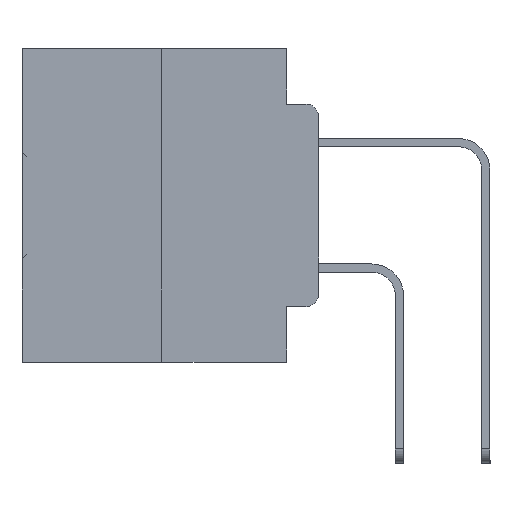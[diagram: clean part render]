
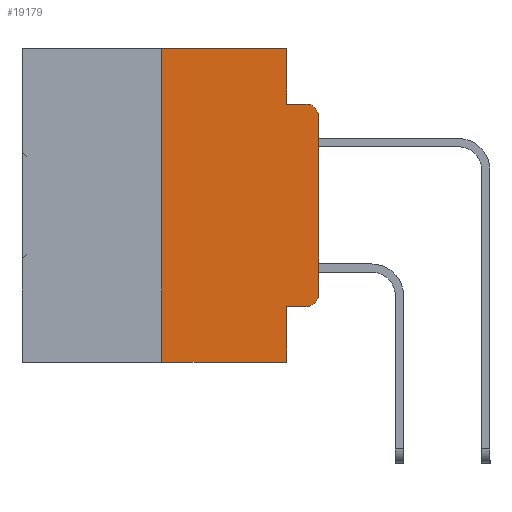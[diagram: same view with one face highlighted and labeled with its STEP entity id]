
A CAD part, left-side view. The second image highlights one B-rep face of the part: STEP entity #19179.
In plain terms, the highlighted planar face has unit normal (-1, 0, 0).
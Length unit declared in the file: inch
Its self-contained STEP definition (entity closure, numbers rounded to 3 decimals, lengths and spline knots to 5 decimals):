
#192 = ORIENTED_EDGE ( 'NONE', *, *, #10469, .T. ) ;
#581 = DIRECTION ( 'NONE',  ( 0., 0., -1. ) ) ;
#603 = ORIENTED_EDGE ( 'NONE', *, *, #27473, .F. ) ;
#792 = VECTOR ( 'NONE', #25249, 39.37008 ) ;
#964 = EDGE_CURVE ( 'NONE', #31384, #4274, #8654, .T. ) ;
#2047 = CARTESIAN_POINT ( 'NONE',  ( 0., 0.473, 0. ) ) ;
#2244 = CARTESIAN_POINT ( 'NONE',  ( 0., 0.473, 0. ) ) ;
#3590 = CARTESIAN_POINT ( 'NONE',  ( 0., 0., -0.3915 ) ) ;
#4274 = VERTEX_POINT ( 'NONE', #27666 ) ;
#4301 = AXIS2_PLACEMENT_3D ( 'NONE', #8759, #27886, #11510 ) ;
#4470 = CARTESIAN_POINT ( 'NONE',  ( 0., 0., 0. ) ) ;
#5002 = DIRECTION ( 'NONE',  ( 0., 0., -1. ) ) ;
#5069 = VERTEX_POINT ( 'NONE', #6417 ) ;
#6417 = CARTESIAN_POINT ( 'NONE',  ( 0., 0., -0.1085 ) ) ;
#7457 = CARTESIAN_POINT ( 'NONE',  ( 0., 0.051, 0. ) ) ;
#7655 = PLANE ( 'NONE',  #8157 ) ;
#8157 = AXIS2_PLACEMENT_3D ( 'NONE', #2244, #21437, #5002 ) ;
#8607 = VECTOR ( 'NONE', #19148, 39.37008 ) ;
#8654 = LINE ( 'NONE', #16856, #23241 ) ;
#8759 = CARTESIAN_POINT ( 'NONE',  ( 0., 0.02, -0.1085 ) ) ;
#9177 = LINE ( 'NONE', #33287, #22912 ) ;
#9994 = VECTOR ( 'NONE', #12510, 39.37008 ) ;
#10026 = ORIENTED_EDGE ( 'NONE', *, *, #31907, .T. ) ;
#10469 = EDGE_CURVE ( 'NONE', #33555, #27536, #14412, .T. ) ;
#10687 = CARTESIAN_POINT ( 'NONE',  ( 0., 0.25, 0. ) ) ;
#11510 = DIRECTION ( 'NONE',  ( 0., 0., -1. ) ) ;
#11627 = CARTESIAN_POINT ( 'NONE',  ( 0., 0.051, -0.4115 ) ) ;
#12165 = EDGE_CURVE ( 'NONE', #5069, #17493, #23960, .T. ) ;
#12510 = DIRECTION ( 'NONE',  ( 0., 0., 1. ) ) ;
#12594 = DIRECTION ( 'NONE',  ( -1., 0., 0. ) ) ;
#13788 = DIRECTION ( 'NONE',  ( 0., 0., -1. ) ) ;
#13917 = AXIS2_PLACEMENT_3D ( 'NONE', #28972, #12594, #31649 ) ;
#14412 = CIRCLE ( 'NONE', #13917, 0.02 ) ;
#15363 = VECTOR ( 'NONE', #19749, 39.37008 ) ;
#16356 = CARTESIAN_POINT ( 'NONE',  ( 0., 0.02, -0.0885 ) ) ;
#16700 = VERTEX_POINT ( 'NONE', #7457 ) ;
#16819 = FACE_OUTER_BOUND ( 'NONE', #20377, .T. ) ;
#16856 = CARTESIAN_POINT ( 'NONE',  ( 0., 0.473, -0.5 ) ) ;
#16872 = ORIENTED_EDGE ( 'NONE', *, *, #31974, .F. ) ;
#16901 = EDGE_CURVE ( 'NONE', #16700, #27307, #29192, .T. ) ;
#17063 = LINE ( 'NONE', #11627, #15363 ) ;
#17280 = VERTEX_POINT ( 'NONE', #26335 ) ;
#17318 = ORIENTED_EDGE ( 'NONE', *, *, #20610, .F. ) ;
#17493 = VERTEX_POINT ( 'NONE', #16356 ) ;
#19148 = DIRECTION ( 'NONE',  ( 0., 0., 1. ) ) ;
#19179 = ADVANCED_FACE ( 'NONE', ( #16819 ), #7655, .F. ) ;
#19429 = ORIENTED_EDGE ( 'NONE', *, *, #12165, .T. ) ;
#19490 = ORIENTED_EDGE ( 'NONE', *, *, #21764, .T. ) ;
#19749 = DIRECTION ( 'NONE',  ( 0., -1., 0. ) ) ;
#19907 = ORIENTED_EDGE ( 'NONE', *, *, #964, .T. ) ;
#20377 = EDGE_LOOP ( 'NONE', ( #10026, #19429, #26325, #25924, #16872, #17318, #19907, #603, #19490, #192 ) ) ;
#20544 = CARTESIAN_POINT ( 'NONE',  ( 0., 0.25, 0. ) ) ;
#20610 = EDGE_CURVE ( 'NONE', #31384, #27333, #30412, .T. ) ;
#21304 = EDGE_CURVE ( 'NONE', #27307, #17493, #22713, .T. ) ;
#21437 = DIRECTION ( 'NONE',  ( 1., 0., 0. ) ) ;
#21759 = CARTESIAN_POINT ( 'NONE',  ( 0., 0.02, -0.4115 ) ) ;
#21764 = EDGE_CURVE ( 'NONE', #17280, #33555, #17063, .T. ) ;
#21995 = VECTOR ( 'NONE', #26740, 39.37008 ) ;
#22499 = CARTESIAN_POINT ( 'NONE',  ( 0., 0.051, -0.0885 ) ) ;
#22713 = LINE ( 'NONE', #22499, #792 ) ;
#22912 = VECTOR ( 'NONE', #581, 39.37008 ) ;
#23241 = VECTOR ( 'NONE', #27413, 39.37008 ) ;
#23960 = CIRCLE ( 'NONE', #4301, 0.02 ) ;
#25249 = DIRECTION ( 'NONE',  ( 0., -1., 0. ) ) ;
#25442 = LINE ( 'NONE', #4470, #9994 ) ;
#25924 = ORIENTED_EDGE ( 'NONE', *, *, #16901, .F. ) ;
#26325 = ORIENTED_EDGE ( 'NONE', *, *, #21304, .F. ) ;
#26335 = CARTESIAN_POINT ( 'NONE',  ( 0., 0.051, -0.4115 ) ) ;
#26740 = DIRECTION ( 'NONE',  ( 0., -1., 0. ) ) ;
#27307 = VERTEX_POINT ( 'NONE', #29704 ) ;
#27333 = VERTEX_POINT ( 'NONE', #10687 ) ;
#27413 = DIRECTION ( 'NONE',  ( 0., -1., 0. ) ) ;
#27473 = EDGE_CURVE ( 'NONE', #17280, #4274, #9177, .T. ) ;
#27536 = VERTEX_POINT ( 'NONE', #3590 ) ;
#27666 = CARTESIAN_POINT ( 'NONE',  ( 0., 0.051, -0.5 ) ) ;
#27886 = DIRECTION ( 'NONE',  ( -1., 0., 0. ) ) ;
#28310 = VECTOR ( 'NONE', #13788, 39.37008 ) ;
#28972 = CARTESIAN_POINT ( 'NONE',  ( 0., 0.02, -0.3915 ) ) ;
#29192 = LINE ( 'NONE', #32808, #28310 ) ;
#29244 = LINE ( 'NONE', #2047, #21995 ) ;
#29704 = CARTESIAN_POINT ( 'NONE',  ( 0., 0.051, -0.0885 ) ) ;
#30412 = LINE ( 'NONE', #20544, #8607 ) ;
#31384 = VERTEX_POINT ( 'NONE', #32189 ) ;
#31649 = DIRECTION ( 'NONE',  ( 0., 0., -1. ) ) ;
#31907 = EDGE_CURVE ( 'NONE', #27536, #5069, #25442, .T. ) ;
#31974 = EDGE_CURVE ( 'NONE', #27333, #16700, #29244, .T. ) ;
#32189 = CARTESIAN_POINT ( 'NONE',  ( 0., 0.25, -0.5 ) ) ;
#32808 = CARTESIAN_POINT ( 'NONE',  ( 0., 0.051, 0. ) ) ;
#33287 = CARTESIAN_POINT ( 'NONE',  ( 0., 0.051, 0. ) ) ;
#33555 = VERTEX_POINT ( 'NONE', #21759 ) ;
